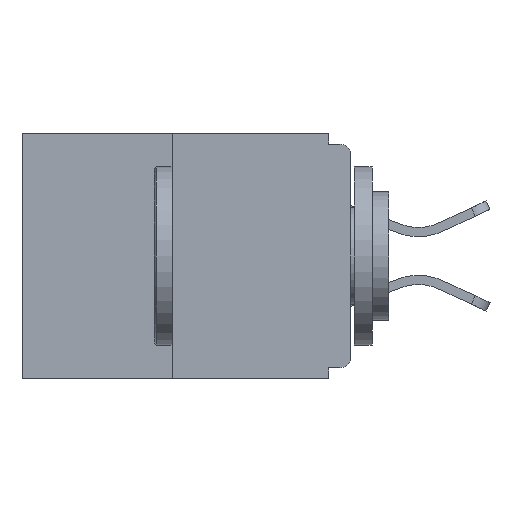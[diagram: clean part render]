
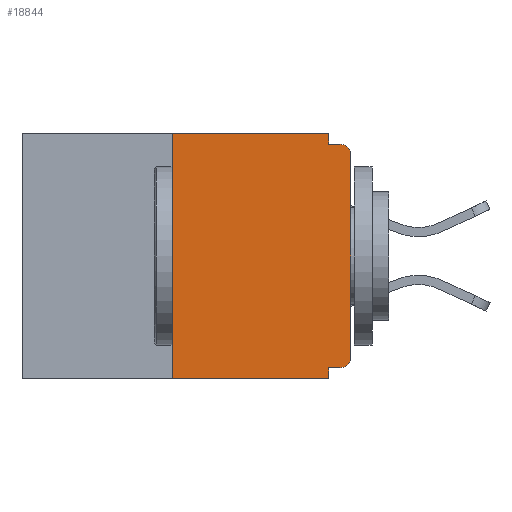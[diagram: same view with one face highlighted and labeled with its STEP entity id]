
A CAD part, left-side view. The second image highlights one B-rep face of the part: STEP entity #18844.
In plain terms, the highlighted planar face has unit normal (-1, 0, 0).
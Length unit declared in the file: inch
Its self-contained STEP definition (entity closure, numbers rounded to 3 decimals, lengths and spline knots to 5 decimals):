
#11 = LINE ( 'NONE', #17763, #7411 ) ;
#124 = CIRCLE ( 'NONE', #14971, 0.015 ) ;
#156 = LINE ( 'NONE', #379, #5371 ) ;
#379 = CARTESIAN_POINT ( 'NONE',  ( 0., 0., -0.328 ) ) ;
#505 = EDGE_CURVE ( 'NONE', #511, #19423, #124, .T. ) ;
#511 = VERTEX_POINT ( 'NONE', #17425 ) ;
#1505 = VECTOR ( 'NONE', #15726, 39.37008 ) ;
#1794 = DIRECTION ( 'NONE',  ( 0., 0., -1. ) ) ;
#1802 = VERTEX_POINT ( 'NONE', #7996 ) ;
#2075 = DIRECTION ( 'NONE',  ( 0., 0., -1. ) ) ;
#2141 = CARTESIAN_POINT ( 'NONE',  ( 0., 0., -0.015 ) ) ;
#2213 = CARTESIAN_POINT ( 'NONE',  ( 0., 0.46, -0.343 ) ) ;
#2379 = VERTEX_POINT ( 'NONE', #11406 ) ;
#3035 = VECTOR ( 'NONE', #9386, 39.37008 ) ;
#3081 = DIRECTION ( 'NONE',  ( -1., 0., 0. ) ) ;
#3932 = LINE ( 'NONE', #19069, #1505 ) ;
#4396 = VECTOR ( 'NONE', #19550, 39.37008 ) ;
#4588 = ORIENTED_EDGE ( 'NONE', *, *, #14825, .F. ) ;
#4809 = CARTESIAN_POINT ( 'NONE',  ( 0., 0.031, -0.015 ) ) ;
#5220 = VECTOR ( 'NONE', #6483, 39.37008 ) ;
#5261 = ORIENTED_EDGE ( 'NONE', *, *, #5491, .F. ) ;
#5326 = EDGE_CURVE ( 'NONE', #19396, #2379, #18402, .T. ) ;
#5371 = VECTOR ( 'NONE', #12425, 39.37008 ) ;
#5380 = ORIENTED_EDGE ( 'NONE', *, *, #8837, .T. ) ;
#5491 = EDGE_CURVE ( 'NONE', #19396, #5832, #7695, .T. ) ;
#5501 = AXIS2_PLACEMENT_3D ( 'NONE', #13975, #19253, #7045 ) ;
#5832 = VERTEX_POINT ( 'NONE', #10032 ) ;
#6359 = VECTOR ( 'NONE', #1794, 39.37008 ) ;
#6483 = DIRECTION ( 'NONE',  ( 0., -1., 0. ) ) ;
#7045 = DIRECTION ( 'NONE',  ( 0., 0., -1. ) ) ;
#7411 = VECTOR ( 'NONE', #21338, 39.37008 ) ;
#7695 = LINE ( 'NONE', #14572, #3035 ) ;
#7996 = CARTESIAN_POINT ( 'NONE',  ( 0., 0., -0.03 ) ) ;
#8128 = ORIENTED_EDGE ( 'NONE', *, *, #5326, .T. ) ;
#8444 = CARTESIAN_POINT ( 'NONE',  ( 0., 0., -0.313 ) ) ;
#8837 = EDGE_CURVE ( 'NONE', #19423, #1802, #3932, .T. ) ;
#8981 = EDGE_CURVE ( 'NONE', #11173, #10806, #19041, .T. ) ;
#9386 = DIRECTION ( 'NONE',  ( 0., 0., 1. ) ) ;
#9710 = EDGE_LOOP ( 'NONE', ( #11776, #5261, #8128, #10844, #4588, #18706, #5380, #13338, #13924, #10593 ) ) ;
#10032 = CARTESIAN_POINT ( 'NONE',  ( 0., 0.25, 0. ) ) ;
#10593 = ORIENTED_EDGE ( 'NONE', *, *, #19515, .F. ) ;
#10732 = DIRECTION ( 'NONE',  ( 1., 0., 0. ) ) ;
#10806 = VERTEX_POINT ( 'NONE', #11809 ) ;
#10815 = CARTESIAN_POINT ( 'NONE',  ( 0., 0.46, 0. ) ) ;
#10844 = ORIENTED_EDGE ( 'NONE', *, *, #21568, .F. ) ;
#11173 = VERTEX_POINT ( 'NONE', #4809 ) ;
#11220 = LINE ( 'NONE', #19706, #5220 ) ;
#11222 = CARTESIAN_POINT ( 'NONE',  ( 0., 0.031, -0.328 ) ) ;
#11406 = CARTESIAN_POINT ( 'NONE',  ( 0., 0.031, -0.343 ) ) ;
#11776 = ORIENTED_EDGE ( 'NONE', *, *, #11788, .F. ) ;
#11788 = EDGE_CURVE ( 'NONE', #5832, #13890, #11220, .T. ) ;
#11809 = CARTESIAN_POINT ( 'NONE',  ( 0., 0.015, -0.015 ) ) ;
#12043 = VERTEX_POINT ( 'NONE', #11222 ) ;
#12415 = LINE ( 'NONE', #15904, #6359 ) ;
#12425 = DIRECTION ( 'NONE',  ( 0., 1., 0. ) ) ;
#12457 = AXIS2_PLACEMENT_3D ( 'NONE', #10815, #10732, #2075 ) ;
#12546 = DIRECTION ( 'NONE',  ( 0., -1., 0. ) ) ;
#13338 = ORIENTED_EDGE ( 'NONE', *, *, #15846, .T. ) ;
#13890 = VERTEX_POINT ( 'NONE', #22535 ) ;
#13924 = ORIENTED_EDGE ( 'NONE', *, *, #8981, .F. ) ;
#13975 = CARTESIAN_POINT ( 'NONE',  ( 0., 0.015, -0.03 ) ) ;
#14572 = CARTESIAN_POINT ( 'NONE',  ( 0., 0.25, 0. ) ) ;
#14575 = PLANE ( 'NONE',  #12457 ) ;
#14825 = EDGE_CURVE ( 'NONE', #511, #12043, #156, .T. ) ;
#14971 = AXIS2_PLACEMENT_3D ( 'NONE', #17264, #3081, #19032 ) ;
#15678 = CARTESIAN_POINT ( 'NONE',  ( 0., 0.25, -0.343 ) ) ;
#15726 = DIRECTION ( 'NONE',  ( 0., 0., 1. ) ) ;
#15846 = EDGE_CURVE ( 'NONE', #1802, #10806, #20719, .T. ) ;
#15904 = CARTESIAN_POINT ( 'NONE',  ( 0., 0.031, 0. ) ) ;
#17264 = CARTESIAN_POINT ( 'NONE',  ( 0., 0.015, -0.313 ) ) ;
#17425 = CARTESIAN_POINT ( 'NONE',  ( 0., 0.015, -0.328 ) ) ;
#17763 = CARTESIAN_POINT ( 'NONE',  ( 0., 0.031, -0.343 ) ) ;
#18402 = LINE ( 'NONE', #2213, #4396 ) ;
#18706 = ORIENTED_EDGE ( 'NONE', *, *, #505, .T. ) ;
#18844 = ADVANCED_FACE ( 'NONE', ( #21802 ), #14575, .F. ) ;
#19032 = DIRECTION ( 'NONE',  ( 0., 0., -1. ) ) ;
#19041 = LINE ( 'NONE', #2141, #20437 ) ;
#19069 = CARTESIAN_POINT ( 'NONE',  ( 0., 0., 0. ) ) ;
#19253 = DIRECTION ( 'NONE',  ( -1., 0., 0. ) ) ;
#19396 = VERTEX_POINT ( 'NONE', #15678 ) ;
#19423 = VERTEX_POINT ( 'NONE', #8444 ) ;
#19515 = EDGE_CURVE ( 'NONE', #13890, #11173, #12415, .T. ) ;
#19550 = DIRECTION ( 'NONE',  ( 0., -1., 0. ) ) ;
#19706 = CARTESIAN_POINT ( 'NONE',  ( 0., 0.46, 0. ) ) ;
#20437 = VECTOR ( 'NONE', #12546, 39.37008 ) ;
#20719 = CIRCLE ( 'NONE', #5501, 0.015 ) ;
#21338 = DIRECTION ( 'NONE',  ( 0., 0., -1. ) ) ;
#21568 = EDGE_CURVE ( 'NONE', #12043, #2379, #11, .T. ) ;
#21802 = FACE_OUTER_BOUND ( 'NONE', #9710, .T. ) ;
#22535 = CARTESIAN_POINT ( 'NONE',  ( 0., 0.031, 0. ) ) ;
